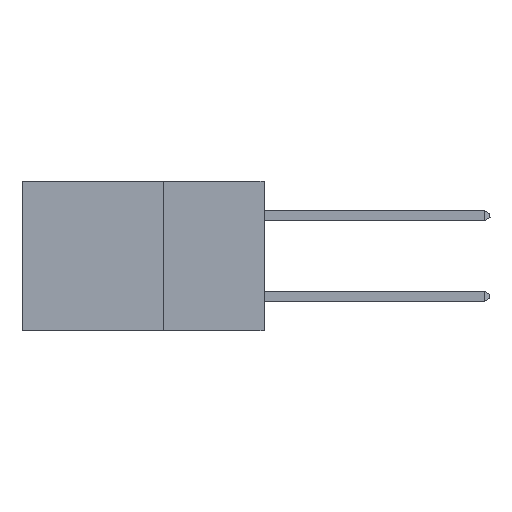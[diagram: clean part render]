
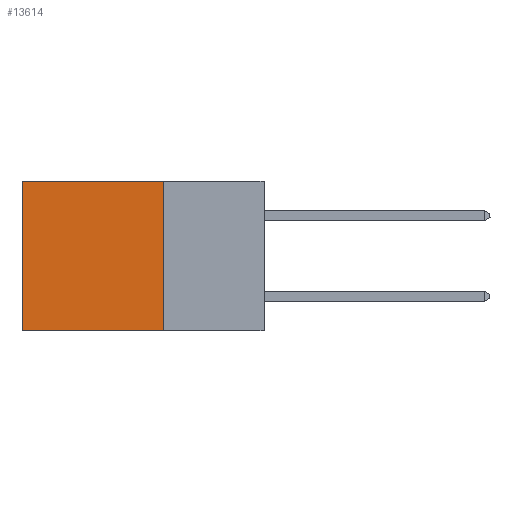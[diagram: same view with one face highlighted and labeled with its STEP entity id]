
A CAD part, left-side view. The second image highlights one B-rep face of the part: STEP entity #13614.
In plain terms, the highlighted planar face has unit normal (-1, 0, 0).
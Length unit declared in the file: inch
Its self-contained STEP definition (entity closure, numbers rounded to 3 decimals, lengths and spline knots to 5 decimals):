
#53 = DIRECTION ( 'NONE',  ( 0., 0., -1. ) ) ;
#61 = DIRECTION ( 'NONE',  ( 0., 0., -1. ) ) ;
#141 = LINE ( 'NONE', #15903, #12688 ) ;
#285 = ORIENTED_EDGE ( 'NONE', *, *, #10734, .T. ) ;
#1279 = PLANE ( 'NONE',  #19101 ) ;
#2835 = VERTEX_POINT ( 'NONE', #11373 ) ;
#2957 = DIRECTION ( 'NONE',  ( 0., 0., -1. ) ) ;
#4395 = EDGE_LOOP ( 'NONE', ( #285, #19706, #8027, #15349 ) ) ;
#6420 = VECTOR ( 'NONE', #61, 39.37008 ) ;
#6706 = CARTESIAN_POINT ( 'NONE',  ( 0.298, 0.6, 0. ) ) ;
#6945 = EDGE_CURVE ( 'NONE', #19138, #9151, #12998, .T. ) ;
#7785 = CARTESIAN_POINT ( 'NONE',  ( 0.298, 0.25, 0. ) ) ;
#8027 = ORIENTED_EDGE ( 'NONE', *, *, #6945, .F. ) ;
#8764 = VECTOR ( 'NONE', #53, 39.37008 ) ;
#9151 = VERTEX_POINT ( 'NONE', #9156 ) ;
#9156 = CARTESIAN_POINT ( 'NONE',  ( 0.298, 0.25, -0.37 ) ) ;
#9595 = FACE_OUTER_BOUND ( 'NONE', #4395, .T. ) ;
#9857 = EDGE_CURVE ( 'NONE', #19138, #13165, #16110, .T. ) ;
#10734 = EDGE_CURVE ( 'NONE', #13165, #2835, #19189, .T. ) ;
#11135 = CARTESIAN_POINT ( 'NONE',  ( 0.298, 0.25, 0. ) ) ;
#11373 = CARTESIAN_POINT ( 'NONE',  ( 0.298, 0.6, -0.37 ) ) ;
#12688 = VECTOR ( 'NONE', #20678, 39.37008 ) ;
#12707 = DIRECTION ( 'NONE',  ( 1., 0., 0. ) ) ;
#12998 = LINE ( 'NONE', #17868, #8764 ) ;
#13165 = VERTEX_POINT ( 'NONE', #6706 ) ;
#13614 = ADVANCED_FACE ( 'NONE', ( #9595 ), #1279, .F. ) ;
#14731 = CARTESIAN_POINT ( 'NONE',  ( 0.298, 0.6, 0. ) ) ;
#15349 = ORIENTED_EDGE ( 'NONE', *, *, #9857, .T. ) ;
#15903 = CARTESIAN_POINT ( 'NONE',  ( 0.298, 0.25, -0.37 ) ) ;
#16110 = LINE ( 'NONE', #7785, #20385 ) ;
#16605 = EDGE_CURVE ( 'NONE', #9151, #2835, #141, .T. ) ;
#17868 = CARTESIAN_POINT ( 'NONE',  ( 0.298, 0.25, 0. ) ) ;
#18950 = CARTESIAN_POINT ( 'NONE',  ( 0.298, 0.25, 0. ) ) ;
#18979 = DIRECTION ( 'NONE',  ( 0., 1., 0. ) ) ;
#19101 = AXIS2_PLACEMENT_3D ( 'NONE', #11135, #12707, #2957 ) ;
#19138 = VERTEX_POINT ( 'NONE', #18950 ) ;
#19189 = LINE ( 'NONE', #14731, #6420 ) ;
#19706 = ORIENTED_EDGE ( 'NONE', *, *, #16605, .F. ) ;
#20385 = VECTOR ( 'NONE', #18979, 39.37008 ) ;
#20678 = DIRECTION ( 'NONE',  ( 0., 1., 0. ) ) ;
